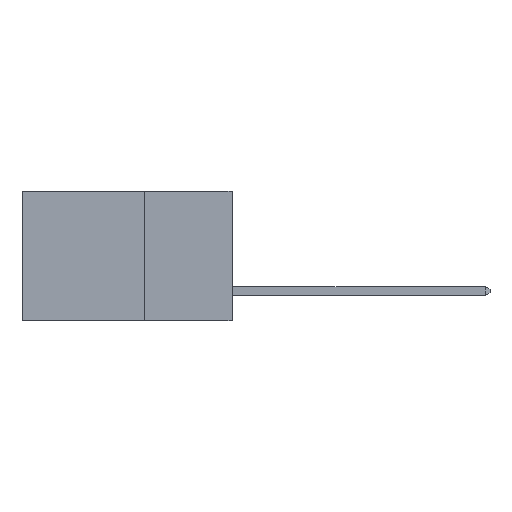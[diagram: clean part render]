
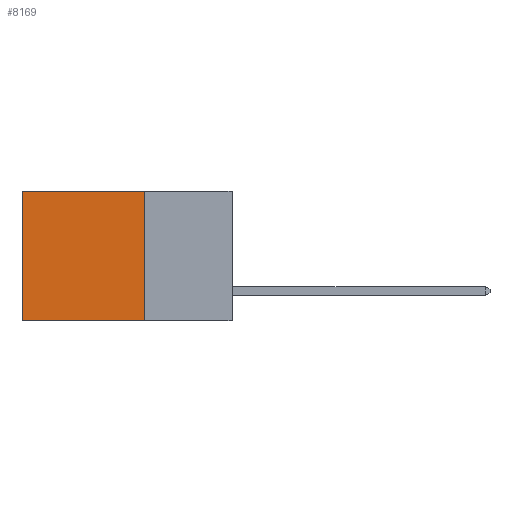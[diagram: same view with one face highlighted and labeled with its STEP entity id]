
A CAD part, left-side view. The second image highlights one B-rep face of the part: STEP entity #8169.
In plain terms, the highlighted planar face has unit normal (-1, 0, 0).
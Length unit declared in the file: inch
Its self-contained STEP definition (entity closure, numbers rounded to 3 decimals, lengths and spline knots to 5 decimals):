
#1602 = DIRECTION ( 'NONE',  ( 0., 1., 0. ) ) ;
#1610 = CARTESIAN_POINT ( 'NONE',  ( 0.2875, 0.6, 0. ) ) ;
#1946 = ORIENTED_EDGE ( 'NONE', *, *, #5639, .T. ) ;
#2141 = CARTESIAN_POINT ( 'NONE',  ( 0.2875, 0.6, 0. ) ) ;
#2213 = EDGE_CURVE ( 'NONE', #12594, #2223, #22743, .T. ) ;
#2223 = VERTEX_POINT ( 'NONE', #21490 ) ;
#2697 = ORIENTED_EDGE ( 'NONE', *, *, #2213, .F. ) ;
#4054 = VECTOR ( 'NONE', #22640, 39.37008 ) ;
#4251 = CARTESIAN_POINT ( 'NONE',  ( 0.2875, 0.6, -0.37 ) ) ;
#4810 = LINE ( 'NONE', #1610, #4054 ) ;
#5639 = EDGE_CURVE ( 'NONE', #12594, #25094, #5744, .T. ) ;
#5744 = LINE ( 'NONE', #22633, #23612 ) ;
#7310 = VECTOR ( 'NONE', #19923, 39.37008 ) ;
#8169 = ADVANCED_FACE ( 'NONE', ( #25303 ), #21524, .F. ) ;
#9797 = CARTESIAN_POINT ( 'NONE',  ( 0.2875, 0.25, 0. ) ) ;
#9855 = EDGE_CURVE ( 'NONE', #2223, #15961, #25909, .T. ) ;
#9933 = DIRECTION ( 'NONE',  ( 0., 0., -1. ) ) ;
#10361 = EDGE_LOOP ( 'NONE', ( #17241, #16326, #2697, #1946 ) ) ;
#12594 = VERTEX_POINT ( 'NONE', #29979 ) ;
#13539 = AXIS2_PLACEMENT_3D ( 'NONE', #16904, #23882, #9933 ) ;
#15961 = VERTEX_POINT ( 'NONE', #4251 ) ;
#16326 = ORIENTED_EDGE ( 'NONE', *, *, #9855, .F. ) ;
#16580 = VECTOR ( 'NONE', #19164, 39.37008 ) ;
#16904 = CARTESIAN_POINT ( 'NONE',  ( 0.2875, 0.25, 0. ) ) ;
#17169 = EDGE_CURVE ( 'NONE', #25094, #15961, #4810, .T. ) ;
#17241 = ORIENTED_EDGE ( 'NONE', *, *, #17169, .T. ) ;
#17605 = CARTESIAN_POINT ( 'NONE',  ( 0.2875, 0.25, -0.37 ) ) ;
#19164 = DIRECTION ( 'NONE',  ( 0., 0., -1. ) ) ;
#19923 = DIRECTION ( 'NONE',  ( 0., 1., 0. ) ) ;
#21490 = CARTESIAN_POINT ( 'NONE',  ( 0.2875, 0.25, -0.37 ) ) ;
#21524 = PLANE ( 'NONE',  #13539 ) ;
#22633 = CARTESIAN_POINT ( 'NONE',  ( 0.2875, 0.25, 0. ) ) ;
#22640 = DIRECTION ( 'NONE',  ( 0., 0., -1. ) ) ;
#22743 = LINE ( 'NONE', #9797, #16580 ) ;
#23612 = VECTOR ( 'NONE', #1602, 39.37008 ) ;
#23882 = DIRECTION ( 'NONE',  ( 1., 0., 0. ) ) ;
#25094 = VERTEX_POINT ( 'NONE', #2141 ) ;
#25303 = FACE_OUTER_BOUND ( 'NONE', #10361, .T. ) ;
#25909 = LINE ( 'NONE', #17605, #7310 ) ;
#29979 = CARTESIAN_POINT ( 'NONE',  ( 0.2875, 0.25, 0. ) ) ;
